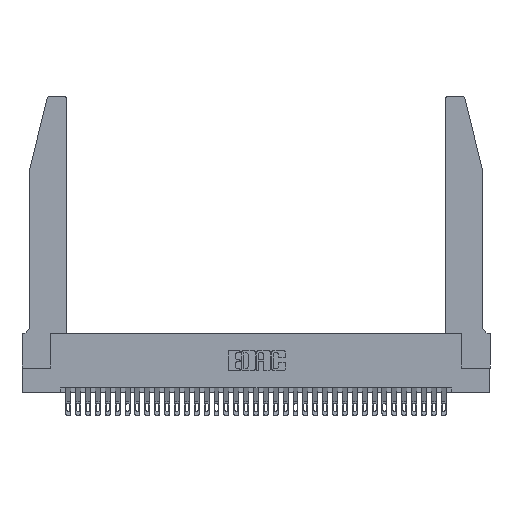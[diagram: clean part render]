
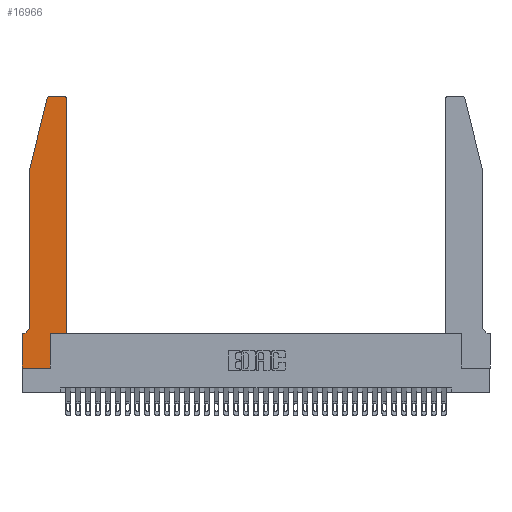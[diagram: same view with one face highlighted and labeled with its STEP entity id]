
A CAD part, top view. The second image highlights one B-rep face of the part: STEP entity #16966.
In plain terms, the highlighted planar face has unit normal (0, 0, 1).
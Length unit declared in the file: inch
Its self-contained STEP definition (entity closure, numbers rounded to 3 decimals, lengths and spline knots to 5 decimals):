
#103 = VERTEX_POINT ( 'NONE', #20168 ) ;
#1076 = CARTESIAN_POINT ( 'NONE',  ( 0., 0., 0.37 ) ) ;
#1088 = CIRCLE ( 'NONE', #21564, 0.07 ) ;
#1283 = CARTESIAN_POINT ( 'NONE',  ( 0.4505, 2.72, 0.37 ) ) ;
#1322 = LINE ( 'NONE', #11402, #15535 ) ;
#1356 = VERTEX_POINT ( 'NONE', #11065 ) ;
#2047 = DIRECTION ( 'NONE',  ( -1., 0., 0. ) ) ;
#2431 = EDGE_CURVE ( 'NONE', #27613, #22327, #27801, .T. ) ;
#2836 = EDGE_CURVE ( 'NONE', #31729, #7500, #26744, .T. ) ;
#2854 = CARTESIAN_POINT ( 'NONE',  ( 0.284, 2.72, 0.37 ) ) ;
#3303 = DIRECTION ( 'NONE',  ( 1., 0., 0. ) ) ;
#3385 = DIRECTION ( 'NONE',  ( 0., -1., 0. ) ) ;
#3387 = CARTESIAN_POINT ( 'NONE',  ( 0.4205, 2.75, 0.37 ) ) ;
#3418 = DIRECTION ( 'NONE',  ( 0., 0., -1. ) ) ;
#3665 = CARTESIAN_POINT ( 'NONE',  ( 0.4205, 2.72, 0.37 ) ) ;
#4521 = EDGE_LOOP ( 'NONE', ( #16039, #18687, #23054, #5016, #34573, #23497, #10366, #22220, #31202, #25646, #20955, #16111 ) ) ;
#4981 = EDGE_CURVE ( 'NONE', #1356, #33178, #31742, .T. ) ;
#5016 = ORIENTED_EDGE ( 'NONE', *, *, #21035, .T. ) ;
#5169 = CARTESIAN_POINT ( 'NONE',  ( 0.4505, 0.35, 0.37 ) ) ;
#5240 = VECTOR ( 'NONE', #19032, 39.37008 ) ;
#5746 = DIRECTION ( 'NONE',  ( 1., 0., 0. ) ) ;
#6147 = DIRECTION ( 'NONE',  ( -0.239, -0.971, 0. ) ) ;
#6564 = DIRECTION ( 'NONE',  ( 1., 0., 0. ) ) ;
#7151 = CARTESIAN_POINT ( 'NONE',  ( 0., 0.35, 0.37 ) ) ;
#7500 = VERTEX_POINT ( 'NONE', #27332 ) ;
#7507 = CARTESIAN_POINT ( 'NONE',  ( 0.284, 2.75, 0.37 ) ) ;
#8380 = EDGE_CURVE ( 'NONE', #29774, #1356, #1322, .T. ) ;
#8827 = EDGE_CURVE ( 'NONE', #33178, #14257, #28097, .T. ) ;
#9617 = VECTOR ( 'NONE', #14609, 39.37008 ) ;
#9627 = LINE ( 'NONE', #28451, #30890 ) ;
#9640 = CARTESIAN_POINT ( 'NONE',  ( 0.2605, 2.75, 0.37 ) ) ;
#9692 = VECTOR ( 'NONE', #2047, 39.37008 ) ;
#10366 = ORIENTED_EDGE ( 'NONE', *, *, #30119, .T. ) ;
#10540 = CARTESIAN_POINT ( 'NONE',  ( 0.0755, 0.35, 0.37 ) ) ;
#11065 = CARTESIAN_POINT ( 'NONE',  ( 0.2865, 0., 0.37 ) ) ;
#11402 = CARTESIAN_POINT ( 'NONE',  ( 0., 0., 0.37 ) ) ;
#11921 = AXIS2_PLACEMENT_3D ( 'NONE', #2854, #22583, #5746 ) ;
#12099 = VERTEX_POINT ( 'NONE', #1283 ) ;
#12729 = VERTEX_POINT ( 'NONE', #7151 ) ;
#12772 = LINE ( 'NONE', #32694, #5240 ) ;
#12866 = EDGE_CURVE ( 'NONE', #15426, #103, #1088, .T. ) ;
#12918 = EDGE_CURVE ( 'NONE', #12099, #27613, #30872, .T. ) ;
#13083 = VECTOR ( 'NONE', #31817, 39.37008 ) ;
#14257 = VERTEX_POINT ( 'NONE', #14849 ) ;
#14609 = DIRECTION ( 'NONE',  ( 0., 1., 0. ) ) ;
#14849 = CARTESIAN_POINT ( 'NONE',  ( 0.4505, 0.35, 0.37 ) ) ;
#15426 = VERTEX_POINT ( 'NONE', #25702 ) ;
#15535 = VECTOR ( 'NONE', #22646, 39.37008 ) ;
#16039 = ORIENTED_EDGE ( 'NONE', *, *, #2431, .T. ) ;
#16111 = ORIENTED_EDGE ( 'NONE', *, *, #12918, .T. ) ;
#16966 = ADVANCED_FACE ( 'NONE', ( #32453 ), #33871, .T. ) ;
#17417 = CARTESIAN_POINT ( 'NONE',  ( 0., 0.35, 0.37 ) ) ;
#18687 = ORIENTED_EDGE ( 'NONE', *, *, #22543, .T. ) ;
#19032 = DIRECTION ( 'NONE',  ( 0., 1., 0. ) ) ;
#19454 = VECTOR ( 'NONE', #6147, 39.37008 ) ;
#19967 = VECTOR ( 'NONE', #24889, 39.37008 ) ;
#20168 = CARTESIAN_POINT ( 'NONE',  ( 0.0055, 0.35, 0.37 ) ) ;
#20228 = EDGE_CURVE ( 'NONE', #14257, #12099, #12772, .T. ) ;
#20255 = DIRECTION ( 'NONE',  ( 0., 0., 1. ) ) ;
#20365 = CARTESIAN_POINT ( 'NONE',  ( 0.0055, 0.42, 0.37 ) ) ;
#20456 = VECTOR ( 'NONE', #20772, 39.37008 ) ;
#20772 = DIRECTION ( 'NONE',  ( 0., -1., 0. ) ) ;
#20955 = ORIENTED_EDGE ( 'NONE', *, *, #20228, .T. ) ;
#21035 = EDGE_CURVE ( 'NONE', #7500, #15426, #9627, .T. ) ;
#21312 = LINE ( 'NONE', #1076, #20456 ) ;
#21564 = AXIS2_PLACEMENT_3D ( 'NONE', #20365, #3418, #23128 ) ;
#22220 = ORIENTED_EDGE ( 'NONE', *, *, #8380, .T. ) ;
#22327 = VERTEX_POINT ( 'NONE', #7507 ) ;
#22543 = EDGE_CURVE ( 'NONE', #22327, #31729, #23659, .T. ) ;
#22583 = DIRECTION ( 'NONE',  ( 0., 0., 1. ) ) ;
#22646 = DIRECTION ( 'NONE',  ( 1., 0., 0. ) ) ;
#22961 = CARTESIAN_POINT ( 'NONE',  ( 0.0755, 2., 0.37 ) ) ;
#22975 = CARTESIAN_POINT ( 'NONE',  ( 0.25487, 2.72718, 0.37 ) ) ;
#23054 = ORIENTED_EDGE ( 'NONE', *, *, #2836, .T. ) ;
#23128 = DIRECTION ( 'NONE',  ( -1., 0., 0. ) ) ;
#23364 = DIRECTION ( 'NONE',  ( 0., 0., 1. ) ) ;
#23497 = ORIENTED_EDGE ( 'NONE', *, *, #32720, .T. ) ;
#23659 = CIRCLE ( 'NONE', #11921, 0.03 ) ;
#24889 = DIRECTION ( 'NONE',  ( 1., 0., 0. ) ) ;
#25393 = LINE ( 'NONE', #10540, #9692 ) ;
#25646 = ORIENTED_EDGE ( 'NONE', *, *, #8827, .T. ) ;
#25702 = CARTESIAN_POINT ( 'NONE',  ( 0.0755, 0.42, 0.37 ) ) ;
#26744 = LINE ( 'NONE', #22961, #19454 ) ;
#27332 = CARTESIAN_POINT ( 'NONE',  ( 0.0755, 2., 0.37 ) ) ;
#27613 = VERTEX_POINT ( 'NONE', #3387 ) ;
#27801 = LINE ( 'NONE', #9640, #13083 ) ;
#28030 = AXIS2_PLACEMENT_3D ( 'NONE', #17417, #20255, #3303 ) ;
#28097 = LINE ( 'NONE', #5169, #19967 ) ;
#28451 = CARTESIAN_POINT ( 'NONE',  ( 0.0755, 2., 0.37 ) ) ;
#29774 = VERTEX_POINT ( 'NONE', #30104 ) ;
#30104 = CARTESIAN_POINT ( 'NONE',  ( 0., 0., 0.37 ) ) ;
#30119 = EDGE_CURVE ( 'NONE', #12729, #29774, #21312, .T. ) ;
#30726 = AXIS2_PLACEMENT_3D ( 'NONE', #3665, #23364, #6564 ) ;
#30872 = CIRCLE ( 'NONE', #30726, 0.03 ) ;
#30890 = VECTOR ( 'NONE', #3385, 39.37008 ) ;
#31202 = ORIENTED_EDGE ( 'NONE', *, *, #4981, .T. ) ;
#31729 = VERTEX_POINT ( 'NONE', #22975 ) ;
#31742 = LINE ( 'NONE', #33898, #9617 ) ;
#31817 = DIRECTION ( 'NONE',  ( -1., 0., 0. ) ) ;
#31833 = CARTESIAN_POINT ( 'NONE',  ( 0.2865, 0.35, 0.37 ) ) ;
#32453 = FACE_OUTER_BOUND ( 'NONE', #4521, .T. ) ;
#32694 = CARTESIAN_POINT ( 'NONE',  ( 0.4505, 0.35, 0.37 ) ) ;
#32720 = EDGE_CURVE ( 'NONE', #103, #12729, #25393, .T. ) ;
#33178 = VERTEX_POINT ( 'NONE', #31833 ) ;
#33871 = PLANE ( 'NONE',  #28030 ) ;
#33898 = CARTESIAN_POINT ( 'NONE',  ( 0.2865, 0.35, 0.37 ) ) ;
#34573 = ORIENTED_EDGE ( 'NONE', *, *, #12866, .T. ) ;
